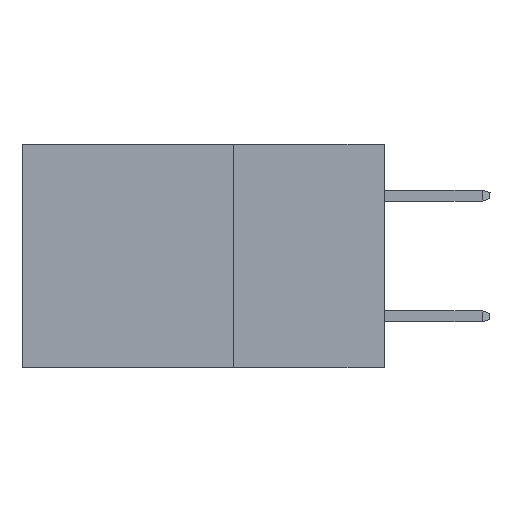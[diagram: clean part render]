
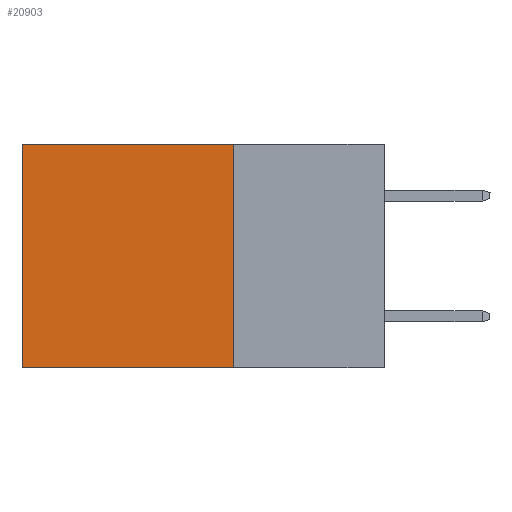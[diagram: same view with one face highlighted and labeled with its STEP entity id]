
A CAD part, left-side view. The second image highlights one B-rep face of the part: STEP entity #20903.
In plain terms, the highlighted planar face has unit normal (-1, 0, 0).
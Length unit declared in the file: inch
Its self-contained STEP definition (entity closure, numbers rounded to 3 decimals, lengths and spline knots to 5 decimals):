
#9 = CARTESIAN_POINT ( 'NONE',  ( 0.298, 0.25, 0. ) ) ;
#39 = LINE ( 'NONE', #23331, #31359 ) ;
#1431 = EDGE_LOOP ( 'NONE', ( #31308, #14995, #22857, #9743 ) ) ;
#1952 = CARTESIAN_POINT ( 'NONE',  ( 0.298, 0.25, 0. ) ) ;
#2628 = DIRECTION ( 'NONE',  ( 1., 0., 0. ) ) ;
#3772 = LINE ( 'NONE', #1952, #22739 ) ;
#3997 = EDGE_CURVE ( 'NONE', #15495, #23424, #27042, .T. ) ;
#8529 = CARTESIAN_POINT ( 'NONE',  ( 0.298, 0.25, -0.37 ) ) ;
#8704 = DIRECTION ( 'NONE',  ( 0., 0., -1. ) ) ;
#9743 = ORIENTED_EDGE ( 'NONE', *, *, #20708, .T. ) ;
#10827 = EDGE_CURVE ( 'NONE', #23424, #30997, #13160, .T. ) ;
#11614 = VECTOR ( 'NONE', #31096, 39.37008 ) ;
#11699 = CARTESIAN_POINT ( 'NONE',  ( 0.298, 0.25, -0.37 ) ) ;
#12070 = DIRECTION ( 'NONE',  ( 0., 1., 0. ) ) ;
#13160 = LINE ( 'NONE', #11699, #11614 ) ;
#14995 = ORIENTED_EDGE ( 'NONE', *, *, #10827, .F. ) ;
#15495 = VERTEX_POINT ( 'NONE', #20225 ) ;
#16157 = CARTESIAN_POINT ( 'NONE',  ( 0.298, 0.6, 0. ) ) ;
#18107 = FACE_OUTER_BOUND ( 'NONE', #1431, .T. ) ;
#19481 = CARTESIAN_POINT ( 'NONE',  ( 0.298, 0.6, -0.37 ) ) ;
#20007 = DIRECTION ( 'NONE',  ( 0., 0., -1. ) ) ;
#20225 = CARTESIAN_POINT ( 'NONE',  ( 0.298, 0.25, 0. ) ) ;
#20708 = EDGE_CURVE ( 'NONE', #15495, #29592, #3772, .T. ) ;
#20903 = ADVANCED_FACE ( 'NONE', ( #18107 ), #29667, .F. ) ;
#21356 = VECTOR ( 'NONE', #23846, 39.37008 ) ;
#22739 = VECTOR ( 'NONE', #12070, 39.37008 ) ;
#22857 = ORIENTED_EDGE ( 'NONE', *, *, #3997, .F. ) ;
#23331 = CARTESIAN_POINT ( 'NONE',  ( 0.298, 0.6, 0. ) ) ;
#23424 = VERTEX_POINT ( 'NONE', #8529 ) ;
#23846 = DIRECTION ( 'NONE',  ( 0., 0., -1. ) ) ;
#23883 = CARTESIAN_POINT ( 'NONE',  ( 0.298, 0.25, 0. ) ) ;
#27042 = LINE ( 'NONE', #23883, #21356 ) ;
#29592 = VERTEX_POINT ( 'NONE', #16157 ) ;
#29667 = PLANE ( 'NONE',  #31611 ) ;
#30997 = VERTEX_POINT ( 'NONE', #19481 ) ;
#31096 = DIRECTION ( 'NONE',  ( 0., 1., 0. ) ) ;
#31308 = ORIENTED_EDGE ( 'NONE', *, *, #31933, .T. ) ;
#31359 = VECTOR ( 'NONE', #8704, 39.37008 ) ;
#31611 = AXIS2_PLACEMENT_3D ( 'NONE', #9, #2628, #20007 ) ;
#31933 = EDGE_CURVE ( 'NONE', #29592, #30997, #39, .T. ) ;
